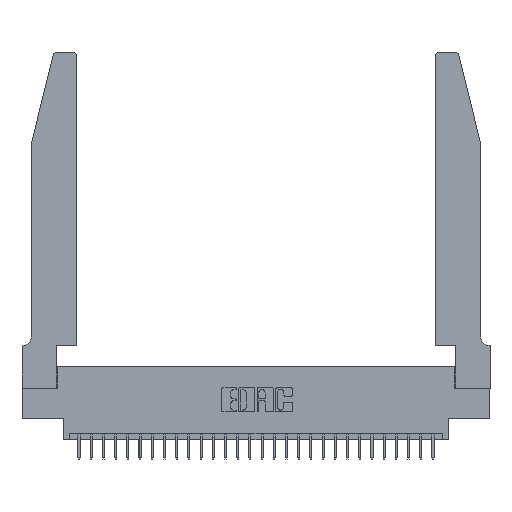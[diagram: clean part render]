
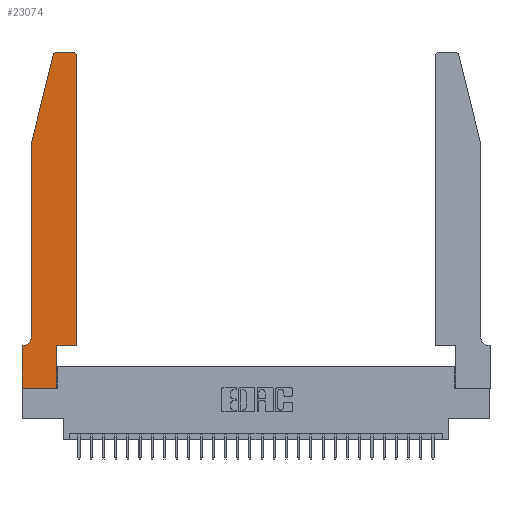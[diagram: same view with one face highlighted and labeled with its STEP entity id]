
A CAD part, top view. The second image highlights one B-rep face of the part: STEP entity #23074.
In plain terms, the highlighted planar face has unit normal (0, 0, 1).
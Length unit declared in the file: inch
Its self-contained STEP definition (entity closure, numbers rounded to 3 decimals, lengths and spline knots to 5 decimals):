
#565 = CARTESIAN_POINT ( 'NONE',  ( 0., 0., 0.37 ) ) ;
#1019 = EDGE_CURVE ( 'NONE', #5562, #5321, #4618, .T. ) ;
#1675 = EDGE_CURVE ( 'NONE', #27260, #4637, #11267, .T. ) ;
#1678 = VERTEX_POINT ( 'NONE', #24961 ) ;
#1782 = CARTESIAN_POINT ( 'NONE',  ( 0.4205, 2.75, 0.37 ) ) ;
#1890 = CARTESIAN_POINT ( 'NONE',  ( 0.4505, 2.72, 0.37 ) ) ;
#2102 = CARTESIAN_POINT ( 'NONE',  ( 0.4205, 2.72, 0.37 ) ) ;
#2171 = EDGE_CURVE ( 'NONE', #5979, #25977, #5271, .T. ) ;
#2314 = AXIS2_PLACEMENT_3D ( 'NONE', #28324, #10038, #26149 ) ;
#2531 = CARTESIAN_POINT ( 'NONE',  ( 0.2865, 0.35, 0.37 ) ) ;
#3666 = ORIENTED_EDGE ( 'NONE', *, *, #15225, .T. ) ;
#4182 = DIRECTION ( 'NONE',  ( 0., -1., 0. ) ) ;
#4538 = DIRECTION ( 'NONE',  ( 1., 0., 0. ) ) ;
#4618 = LINE ( 'NONE', #13588, #10184 ) ;
#4637 = VERTEX_POINT ( 'NONE', #14781 ) ;
#5247 = CARTESIAN_POINT ( 'NONE',  ( 0.0755, 0.42, 0.37 ) ) ;
#5271 = LINE ( 'NONE', #10979, #6772 ) ;
#5321 = VERTEX_POINT ( 'NONE', #5247 ) ;
#5419 = VECTOR ( 'NONE', #9773, 39.37008 ) ;
#5562 = VERTEX_POINT ( 'NONE', #13213 ) ;
#5631 = CARTESIAN_POINT ( 'NONE',  ( 0.0055, 0.35, 0.37 ) ) ;
#5979 = VERTEX_POINT ( 'NONE', #5631 ) ;
#6302 = LINE ( 'NONE', #21829, #11874 ) ;
#6448 = CARTESIAN_POINT ( 'NONE',  ( 0.4505, 0.35, 0.37 ) ) ;
#6524 = CARTESIAN_POINT ( 'NONE',  ( 0.4505, 0.35, 0.37 ) ) ;
#6772 = VECTOR ( 'NONE', #27028, 39.37008 ) ;
#7674 = PLANE ( 'NONE',  #2314 ) ;
#7849 = EDGE_LOOP ( 'NONE', ( #25850, #20345, #3666, #12506, #20138, #21690, #28734, #8133, #29503, #14411, #25820, #26502 ) ) ;
#8133 = ORIENTED_EDGE ( 'NONE', *, *, #18657, .T. ) ;
#8977 = LINE ( 'NONE', #6524, #28067 ) ;
#9773 = DIRECTION ( 'NONE',  ( -0.239, -0.971, 0. ) ) ;
#10038 = DIRECTION ( 'NONE',  ( 0., 0., 1. ) ) ;
#10103 = EDGE_CURVE ( 'NONE', #18701, #24456, #14584, .T. ) ;
#10184 = VECTOR ( 'NONE', #27276, 39.37008 ) ;
#10979 = CARTESIAN_POINT ( 'NONE',  ( 0.0755, 0.35, 0.37 ) ) ;
#11267 = CIRCLE ( 'NONE', #15328, 0.03 ) ;
#11663 = AXIS2_PLACEMENT_3D ( 'NONE', #26103, #12384, #28389 ) ;
#11740 = LINE ( 'NONE', #16799, #5419 ) ;
#11871 = DIRECTION ( 'NONE',  ( 1., 0., 0. ) ) ;
#11874 = VECTOR ( 'NONE', #24131, 39.37008 ) ;
#12384 = DIRECTION ( 'NONE',  ( 0., 0., -1. ) ) ;
#12506 = ORIENTED_EDGE ( 'NONE', *, *, #1019, .T. ) ;
#12676 = VERTEX_POINT ( 'NONE', #1782 ) ;
#12732 = EDGE_CURVE ( 'NONE', #18196, #12676, #19440, .T. ) ;
#13213 = CARTESIAN_POINT ( 'NONE',  ( 0.0755, 2., 0.37 ) ) ;
#13548 = DIRECTION ( 'NONE',  ( 0., 0., 1. ) ) ;
#13565 = LINE ( 'NONE', #15910, #18240 ) ;
#13588 = CARTESIAN_POINT ( 'NONE',  ( 0.0755, 2., 0.37 ) ) ;
#14411 = ORIENTED_EDGE ( 'NONE', *, *, #20731, .T. ) ;
#14584 = LINE ( 'NONE', #2531, #20663 ) ;
#14781 = CARTESIAN_POINT ( 'NONE',  ( 0.25487, 2.72718, 0.37 ) ) ;
#14973 = EDGE_CURVE ( 'NONE', #25977, #19482, #13565, .T. ) ;
#15225 = EDGE_CURVE ( 'NONE', #4637, #5562, #11740, .T. ) ;
#15328 = AXIS2_PLACEMENT_3D ( 'NONE', #27241, #13548, #29543 ) ;
#15631 = LINE ( 'NONE', #6448, #27053 ) ;
#15910 = CARTESIAN_POINT ( 'NONE',  ( 0., 0., 0.37 ) ) ;
#16799 = CARTESIAN_POINT ( 'NONE',  ( 0.0755, 2., 0.37 ) ) ;
#18112 = CARTESIAN_POINT ( 'NONE',  ( 0.284, 2.75, 0.37 ) ) ;
#18196 = VERTEX_POINT ( 'NONE', #1890 ) ;
#18240 = VECTOR ( 'NONE', #4182, 39.37008 ) ;
#18539 = DIRECTION ( 'NONE',  ( 0., 0., 1. ) ) ;
#18593 = FACE_OUTER_BOUND ( 'NONE', #7849, .T. ) ;
#18657 = EDGE_CURVE ( 'NONE', #19482, #18701, #21069, .T. ) ;
#18701 = VERTEX_POINT ( 'NONE', #25707 ) ;
#19111 = CARTESIAN_POINT ( 'NONE',  ( 0.2865, 0.35, 0.37 ) ) ;
#19440 = CIRCLE ( 'NONE', #25650, 0.03 ) ;
#19482 = VERTEX_POINT ( 'NONE', #565 ) ;
#20138 = ORIENTED_EDGE ( 'NONE', *, *, #29937, .T. ) ;
#20345 = ORIENTED_EDGE ( 'NONE', *, *, #1675, .T. ) ;
#20451 = DIRECTION ( 'NONE',  ( 0., 1., 0. ) ) ;
#20663 = VECTOR ( 'NONE', #25664, 39.37008 ) ;
#20731 = EDGE_CURVE ( 'NONE', #24456, #1678, #15631, .T. ) ;
#21069 = LINE ( 'NONE', #25608, #27134 ) ;
#21690 = ORIENTED_EDGE ( 'NONE', *, *, #2171, .T. ) ;
#21829 = CARTESIAN_POINT ( 'NONE',  ( 0.2605, 2.75, 0.37 ) ) ;
#23074 = ADVANCED_FACE ( 'NONE', ( #18593 ), #7674, .T. ) ;
#24131 = DIRECTION ( 'NONE',  ( -1., 0., 0. ) ) ;
#24439 = CIRCLE ( 'NONE', #11663, 0.07 ) ;
#24456 = VERTEX_POINT ( 'NONE', #19111 ) ;
#24961 = CARTESIAN_POINT ( 'NONE',  ( 0.4505, 0.35, 0.37 ) ) ;
#24992 = DIRECTION ( 'NONE',  ( 1., 0., 0. ) ) ;
#25608 = CARTESIAN_POINT ( 'NONE',  ( 0., 0., 0.37 ) ) ;
#25650 = AXIS2_PLACEMENT_3D ( 'NONE', #2102, #18539, #4538 ) ;
#25664 = DIRECTION ( 'NONE',  ( 0., 1., 0. ) ) ;
#25707 = CARTESIAN_POINT ( 'NONE',  ( 0.2865, 0., 0.37 ) ) ;
#25820 = ORIENTED_EDGE ( 'NONE', *, *, #28529, .T. ) ;
#25850 = ORIENTED_EDGE ( 'NONE', *, *, #26989, .T. ) ;
#25977 = VERTEX_POINT ( 'NONE', #29508 ) ;
#26103 = CARTESIAN_POINT ( 'NONE',  ( 0.0055, 0.42, 0.37 ) ) ;
#26149 = DIRECTION ( 'NONE',  ( 1., 0., 0. ) ) ;
#26502 = ORIENTED_EDGE ( 'NONE', *, *, #12732, .T. ) ;
#26989 = EDGE_CURVE ( 'NONE', #12676, #27260, #6302, .T. ) ;
#27028 = DIRECTION ( 'NONE',  ( -1., 0., 0. ) ) ;
#27053 = VECTOR ( 'NONE', #24992, 39.37008 ) ;
#27134 = VECTOR ( 'NONE', #11871, 39.37008 ) ;
#27241 = CARTESIAN_POINT ( 'NONE',  ( 0.284, 2.72, 0.37 ) ) ;
#27260 = VERTEX_POINT ( 'NONE', #18112 ) ;
#27276 = DIRECTION ( 'NONE',  ( 0., -1., 0. ) ) ;
#28067 = VECTOR ( 'NONE', #20451, 39.37008 ) ;
#28324 = CARTESIAN_POINT ( 'NONE',  ( 0., 0.35, 0.37 ) ) ;
#28389 = DIRECTION ( 'NONE',  ( -1., 0., 0. ) ) ;
#28529 = EDGE_CURVE ( 'NONE', #1678, #18196, #8977, .T. ) ;
#28734 = ORIENTED_EDGE ( 'NONE', *, *, #14973, .T. ) ;
#29503 = ORIENTED_EDGE ( 'NONE', *, *, #10103, .T. ) ;
#29508 = CARTESIAN_POINT ( 'NONE',  ( 0., 0.35, 0.37 ) ) ;
#29543 = DIRECTION ( 'NONE',  ( 1., 0., 0. ) ) ;
#29937 = EDGE_CURVE ( 'NONE', #5321, #5979, #24439, .T. ) ;
